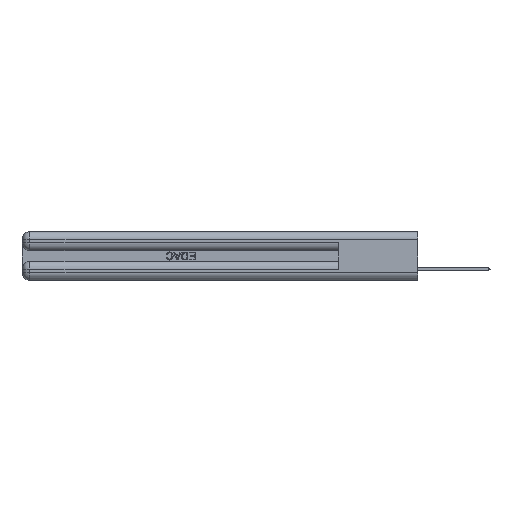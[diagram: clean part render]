
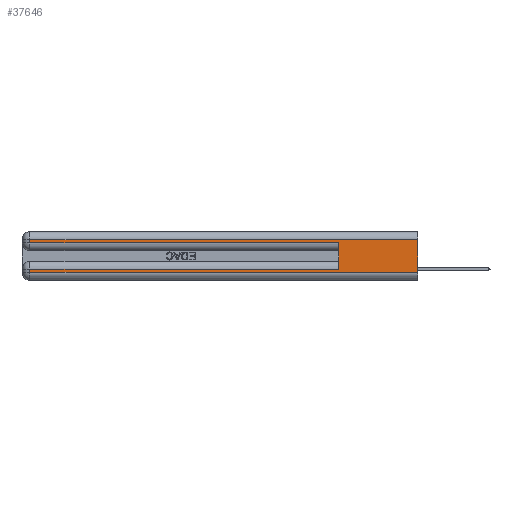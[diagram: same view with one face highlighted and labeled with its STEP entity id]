
A CAD part, left-side view. The second image highlights one B-rep face of the part: STEP entity #37646.
In plain terms, the highlighted planar face has unit normal (-1, 0, 0).
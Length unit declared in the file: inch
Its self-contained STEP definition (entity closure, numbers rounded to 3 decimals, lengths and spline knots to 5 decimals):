
#522 = VERTEX_POINT ( 'NONE', #16854 ) ;
#570 = ORIENTED_EDGE ( 'NONE', *, *, #34433, .F. ) ;
#4710 = EDGE_CURVE ( 'NONE', #31883, #8585, #15290, .T. ) ;
#6712 = ORIENTED_EDGE ( 'NONE', *, *, #4710, .T. ) ;
#7090 = CARTESIAN_POINT ( 'NONE',  ( 0., 2.94, 0.06 ) ) ;
#7914 = CARTESIAN_POINT ( 'NONE',  ( 0., 0., 0.06 ) ) ;
#8538 = EDGE_CURVE ( 'NONE', #52462, #25901, #19419, .T. ) ;
#8554 = VECTOR ( 'NONE', #42840, 39.37008 ) ;
#8585 = VERTEX_POINT ( 'NONE', #26810 ) ;
#8743 = LINE ( 'NONE', #43389, #36284 ) ;
#10734 = EDGE_CURVE ( 'NONE', #52462, #32733, #38936, .T. ) ;
#11301 = CARTESIAN_POINT ( 'NONE',  ( 0., 0., 0.085 ) ) ;
#11510 = DIRECTION ( 'NONE',  ( 0., 0., -1. ) ) ;
#13511 = ORIENTED_EDGE ( 'NONE', *, *, #8538, .T. ) ;
#13561 = AXIS2_PLACEMENT_3D ( 'NONE', #20373, #48807, #11510 ) ;
#13657 = CARTESIAN_POINT ( 'NONE',  ( 0., 2.94, 0.37 ) ) ;
#13738 = EDGE_CURVE ( 'NONE', #8585, #25039, #21611, .T. ) ;
#13971 = EDGE_CURVE ( 'NONE', #25901, #522, #48140, .T. ) ;
#14180 = VECTOR ( 'NONE', #33465, 39.37008 ) ;
#15290 = LINE ( 'NONE', #11301, #39594 ) ;
#16126 = VECTOR ( 'NONE', #37906, 39.37008 ) ;
#16341 = ORIENTED_EDGE ( 'NONE', *, *, #10734, .F. ) ;
#16854 = CARTESIAN_POINT ( 'NONE',  ( 0., 2.94, 0.285 ) ) ;
#17336 = LINE ( 'NONE', #25226, #14180 ) ;
#18151 = DIRECTION ( 'NONE',  ( 0., 0., -1. ) ) ;
#18563 = ORIENTED_EDGE ( 'NONE', *, *, #13738, .T. ) ;
#19419 = LINE ( 'NONE', #30736, #8554 ) ;
#20373 = CARTESIAN_POINT ( 'NONE',  ( 0., 0., 0.37 ) ) ;
#21195 = VECTOR ( 'NONE', #32262, 39.37008 ) ;
#21611 = LINE ( 'NONE', #13657, #30656 ) ;
#21827 = FACE_OUTER_BOUND ( 'NONE', #40519, .T. ) ;
#21913 = DIRECTION ( 'NONE',  ( 0., 0., -1. ) ) ;
#23661 = ORIENTED_EDGE ( 'NONE', *, *, #36791, .T. ) ;
#23720 = CARTESIAN_POINT ( 'NONE',  ( 0., 0.6, 0.285 ) ) ;
#25039 = VERTEX_POINT ( 'NONE', #7090 ) ;
#25226 = CARTESIAN_POINT ( 'NONE',  ( 0., 0., 0.06 ) ) ;
#25501 = VECTOR ( 'NONE', #21913, 39.37008 ) ;
#25901 = VERTEX_POINT ( 'NONE', #44742 ) ;
#26805 = CARTESIAN_POINT ( 'NONE',  ( 0., 0., 0.37 ) ) ;
#26810 = CARTESIAN_POINT ( 'NONE',  ( 0., 2.94, 0.085 ) ) ;
#27573 = DIRECTION ( 'NONE',  ( 0., 1., 0. ) ) ;
#28348 = LINE ( 'NONE', #41983, #16126 ) ;
#30039 = ORIENTED_EDGE ( 'NONE', *, *, #13971, .T. ) ;
#30656 = VECTOR ( 'NONE', #18151, 39.37008 ) ;
#30736 = CARTESIAN_POINT ( 'NONE',  ( 0., 0., 0.31 ) ) ;
#31883 = VERTEX_POINT ( 'NONE', #41081 ) ;
#32087 = PLANE ( 'NONE',  #13561 ) ;
#32262 = DIRECTION ( 'NONE',  ( 0., 0., -1. ) ) ;
#32733 = VERTEX_POINT ( 'NONE', #7914 ) ;
#33465 = DIRECTION ( 'NONE',  ( 0., -1., 0. ) ) ;
#34433 = EDGE_CURVE ( 'NONE', #31883, #44677, #8743, .T. ) ;
#36284 = VECTOR ( 'NONE', #38716, 39.37008 ) ;
#36791 = EDGE_CURVE ( 'NONE', #25039, #32733, #17336, .T. ) ;
#37266 = EDGE_CURVE ( 'NONE', #522, #44677, #28348, .T. ) ;
#37646 = ADVANCED_FACE ( 'NONE', ( #21827 ), #32087, .F. ) ;
#37906 = DIRECTION ( 'NONE',  ( 0., -1., 0. ) ) ;
#38388 = CARTESIAN_POINT ( 'NONE',  ( 0., 0., 0.31 ) ) ;
#38716 = DIRECTION ( 'NONE',  ( 0., 0., 1. ) ) ;
#38936 = LINE ( 'NONE', #26805, #25501 ) ;
#39594 = VECTOR ( 'NONE', #27573, 39.37008 ) ;
#40519 = EDGE_LOOP ( 'NONE', ( #16341, #13511, #30039, #52566, #570, #6712, #18563, #23661 ) ) ;
#41081 = CARTESIAN_POINT ( 'NONE',  ( 0., 0.6, 0.085 ) ) ;
#41983 = CARTESIAN_POINT ( 'NONE',  ( 0., 0., 0.285 ) ) ;
#42840 = DIRECTION ( 'NONE',  ( 0., 1., 0. ) ) ;
#43389 = CARTESIAN_POINT ( 'NONE',  ( 0., 0.6, 0.145 ) ) ;
#44677 = VERTEX_POINT ( 'NONE', #23720 ) ;
#44742 = CARTESIAN_POINT ( 'NONE',  ( 0., 2.94, 0.31 ) ) ;
#48140 = LINE ( 'NONE', #52556, #21195 ) ;
#48807 = DIRECTION ( 'NONE',  ( 1., 0., 0. ) ) ;
#52462 = VERTEX_POINT ( 'NONE', #38388 ) ;
#52556 = CARTESIAN_POINT ( 'NONE',  ( 0., 2.94, 0.37 ) ) ;
#52566 = ORIENTED_EDGE ( 'NONE', *, *, #37266, .T. ) ;
